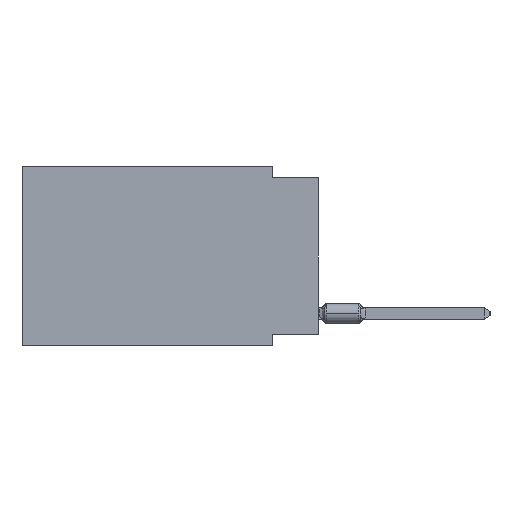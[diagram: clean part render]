
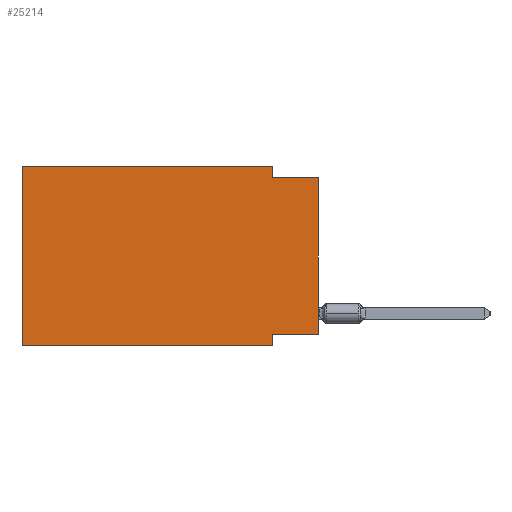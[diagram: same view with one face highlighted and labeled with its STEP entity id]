
A CAD part, left-side view. The second image highlights one B-rep face of the part: STEP entity #25214.
In plain terms, the highlighted planar face has unit normal (-1, 0, 0).
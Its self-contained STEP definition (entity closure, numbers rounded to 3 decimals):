
#36 = EDGE_LOOP ( 'NONE', ( #11561, #22078, #18215, #9656, #17455, #18551, #4143, #16219 ) ) ;
#116 = EDGE_CURVE ( 'NONE', #27284, #23851, #1230, .T. ) ;
#300 = DIRECTION ( 'NONE',  ( 0., 1., 0. ) ) ;
#874 = VECTOR ( 'NONE', #300, 1000. ) ;
#1042 = VECTOR ( 'NONE', #26625, 1000. ) ;
#1230 = LINE ( 'NONE', #34957, #1042 ) ;
#1808 = CARTESIAN_POINT ( 'NONE',  ( 0., 16.383, 0. ) ) ;
#2349 = CARTESIAN_POINT ( 'NONE',  ( 0., 0., -0.635 ) ) ;
#2579 = EDGE_CURVE ( 'NONE', #3895, #27094, #35898, .T. ) ;
#2617 = EDGE_CURVE ( 'NONE', #23851, #28507, #15451, .T. ) ;
#3298 = DIRECTION ( 'NONE',  ( 0., 0., -1. ) ) ;
#3895 = VERTEX_POINT ( 'NONE', #7604 ) ;
#4143 = ORIENTED_EDGE ( 'NONE', *, *, #14070, .F. ) ;
#4233 = CARTESIAN_POINT ( 'NONE',  ( 0., 16.383, 0. ) ) ;
#4673 = CARTESIAN_POINT ( 'NONE',  ( 0., 2.54, -0.635 ) ) ;
#5351 = LINE ( 'NONE', #22815, #6857 ) ;
#5602 = VECTOR ( 'NONE', #24913, 1000. ) ;
#6149 = VERTEX_POINT ( 'NONE', #4673 ) ;
#6512 = DIRECTION ( 'NONE',  ( 1., 0., 0. ) ) ;
#6857 = VECTOR ( 'NONE', #20137, 1000. ) ;
#6868 = DIRECTION ( 'NONE',  ( 0., 0., -1. ) ) ;
#7112 = EDGE_CURVE ( 'NONE', #3895, #37159, #20955, .T. ) ;
#7604 = CARTESIAN_POINT ( 'NONE',  ( 0., 0., -9.271 ) ) ;
#9510 = VECTOR ( 'NONE', #3298, 1000. ) ;
#9539 = PLANE ( 'NONE',  #9850 ) ;
#9656 = ORIENTED_EDGE ( 'NONE', *, *, #2617, .F. ) ;
#9850 = AXIS2_PLACEMENT_3D ( 'NONE', #4233, #6512, #6868 ) ;
#10327 = LINE ( 'NONE', #10512, #25275 ) ;
#10512 = CARTESIAN_POINT ( 'NONE',  ( 0., 16.383, -9.906 ) ) ;
#11561 = ORIENTED_EDGE ( 'NONE', *, *, #2579, .T. ) ;
#12004 = EDGE_CURVE ( 'NONE', #6149, #27094, #21885, .T. ) ;
#14070 = EDGE_CURVE ( 'NONE', #37159, #14658, #32091, .T. ) ;
#14658 = VERTEX_POINT ( 'NONE', #36022 ) ;
#15451 = LINE ( 'NONE', #18291, #22297 ) ;
#15667 = EDGE_CURVE ( 'NONE', #27284, #14658, #10327, .T. ) ;
#15669 = DIRECTION ( 'NONE',  ( 0., -1., 0. ) ) ;
#16219 = ORIENTED_EDGE ( 'NONE', *, *, #7112, .F. ) ;
#17455 = ORIENTED_EDGE ( 'NONE', *, *, #116, .F. ) ;
#18215 = ORIENTED_EDGE ( 'NONE', *, *, #25615, .F. ) ;
#18291 = CARTESIAN_POINT ( 'NONE',  ( 0., 16.383, 0. ) ) ;
#18551 = ORIENTED_EDGE ( 'NONE', *, *, #15667, .T. ) ;
#20137 = DIRECTION ( 'NONE',  ( 0., 0., -1. ) ) ;
#20955 = LINE ( 'NONE', #23790, #874 ) ;
#21529 = CARTESIAN_POINT ( 'NONE',  ( 0., 0., 0. ) ) ;
#21885 = LINE ( 'NONE', #2349, #5602 ) ;
#22078 = ORIENTED_EDGE ( 'NONE', *, *, #12004, .F. ) ;
#22297 = VECTOR ( 'NONE', #32842, 1000. ) ;
#22815 = CARTESIAN_POINT ( 'NONE',  ( 0., 2.54, 0. ) ) ;
#23790 = CARTESIAN_POINT ( 'NONE',  ( 0., 0., -9.271 ) ) ;
#23851 = VERTEX_POINT ( 'NONE', #1808 ) ;
#23864 = CARTESIAN_POINT ( 'NONE',  ( 0., 16.383, -9.906 ) ) ;
#24913 = DIRECTION ( 'NONE',  ( 0., -1., 0. ) ) ;
#25214 = ADVANCED_FACE ( 'NONE', ( #29790 ), #9539, .F. ) ;
#25275 = VECTOR ( 'NONE', #15669, 1000. ) ;
#25418 = CARTESIAN_POINT ( 'NONE',  ( 0., 2.54, 0. ) ) ;
#25615 = EDGE_CURVE ( 'NONE', #28507, #6149, #5351, .T. ) ;
#26625 = DIRECTION ( 'NONE',  ( 0., 0., 1. ) ) ;
#27094 = VERTEX_POINT ( 'NONE', #31796 ) ;
#27284 = VERTEX_POINT ( 'NONE', #23864 ) ;
#28507 = VERTEX_POINT ( 'NONE', #25418 ) ;
#29009 = CARTESIAN_POINT ( 'NONE',  ( 0., 2.54, -9.271 ) ) ;
#29790 = FACE_OUTER_BOUND ( 'NONE', #36, .T. ) ;
#31796 = CARTESIAN_POINT ( 'NONE',  ( 0., 0., -0.635 ) ) ;
#32091 = LINE ( 'NONE', #35150, #9510 ) ;
#32842 = DIRECTION ( 'NONE',  ( 0., -1., 0. ) ) ;
#34957 = CARTESIAN_POINT ( 'NONE',  ( 0., 16.383, 0. ) ) ;
#35150 = CARTESIAN_POINT ( 'NONE',  ( 0., 2.54, -9.906 ) ) ;
#35328 = DIRECTION ( 'NONE',  ( 0., 0., 1. ) ) ;
#35898 = LINE ( 'NONE', #21529, #37421 ) ;
#36022 = CARTESIAN_POINT ( 'NONE',  ( 0., 2.54, -9.906 ) ) ;
#37159 = VERTEX_POINT ( 'NONE', #29009 ) ;
#37421 = VECTOR ( 'NONE', #35328, 1000. ) ;
